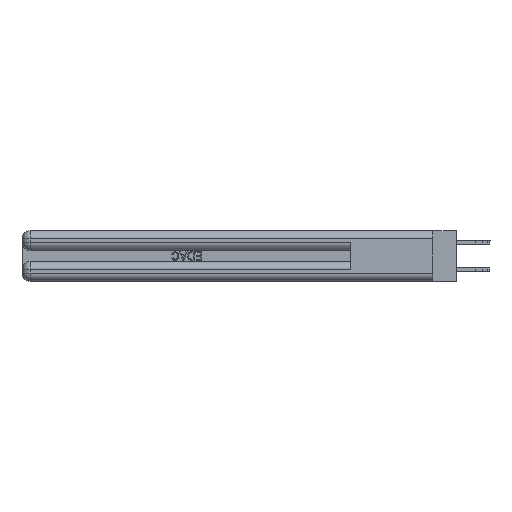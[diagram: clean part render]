
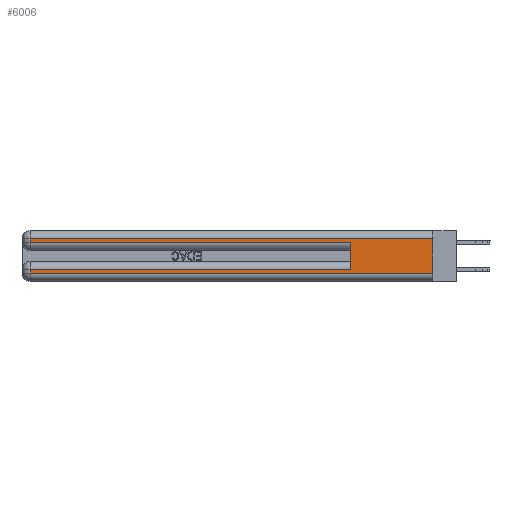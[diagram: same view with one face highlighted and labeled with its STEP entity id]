
A CAD part, left-side view. The second image highlights one B-rep face of the part: STEP entity #6006.
In plain terms, the highlighted planar face has unit normal (-1, 0, 0).
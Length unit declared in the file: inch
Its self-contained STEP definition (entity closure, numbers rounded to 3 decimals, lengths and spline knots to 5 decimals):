
#216 = EDGE_CURVE ( 'NONE', #25626, #29858, #14282, .T. ) ;
#694 = LINE ( 'NONE', #27844, #16419 ) ;
#1438 = VERTEX_POINT ( 'NONE', #34184 ) ;
#1542 = AXIS2_PLACEMENT_3D ( 'NONE', #35377, #20176, #5460 ) ;
#1654 = VERTEX_POINT ( 'NONE', #16338 ) ;
#1658 = CARTESIAN_POINT ( 'NONE',  ( 0., 2.94, 0.37 ) ) ;
#1800 = DIRECTION ( 'NONE',  ( 0., 0., -1. ) ) ;
#2630 = ORIENTED_EDGE ( 'NONE', *, *, #3906, .T. ) ;
#3806 = LINE ( 'NONE', #1658, #14897 ) ;
#3906 = EDGE_CURVE ( 'NONE', #13565, #19742, #37265, .T. ) ;
#4941 = VECTOR ( 'NONE', #24562, 39.37008 ) ;
#5460 = DIRECTION ( 'NONE',  ( 0., 0., -1. ) ) ;
#5715 = VERTEX_POINT ( 'NONE', #21831 ) ;
#5845 = PLANE ( 'NONE',  #1542 ) ;
#6006 = ADVANCED_FACE ( 'NONE', ( #12161 ), #5845, .F. ) ;
#6281 = CARTESIAN_POINT ( 'NONE',  ( 0., 0., 0.285 ) ) ;
#6448 = VECTOR ( 'NONE', #24419, 39.37008 ) ;
#8219 = VECTOR ( 'NONE', #12446, 39.37008 ) ;
#8878 = CARTESIAN_POINT ( 'NONE',  ( 0., 0., 0.06 ) ) ;
#10193 = ORIENTED_EDGE ( 'NONE', *, *, #15186, .T. ) ;
#12161 = FACE_OUTER_BOUND ( 'NONE', #26628, .T. ) ;
#12446 = DIRECTION ( 'NONE',  ( 0., 0., 1. ) ) ;
#13147 = CARTESIAN_POINT ( 'NONE',  ( 0., 0., 0.085 ) ) ;
#13565 = VERTEX_POINT ( 'NONE', #37976 ) ;
#14282 = LINE ( 'NONE', #33454, #6448 ) ;
#14897 = VECTOR ( 'NONE', #1800, 39.37008 ) ;
#15186 = EDGE_CURVE ( 'NONE', #5715, #13565, #16527, .T. ) ;
#15385 = LINE ( 'NONE', #28747, #20918 ) ;
#16338 = CARTESIAN_POINT ( 'NONE',  ( 0., 2.94, 0.085 ) ) ;
#16419 = VECTOR ( 'NONE', #36377, 39.37008 ) ;
#16527 = LINE ( 'NONE', #30966, #19315 ) ;
#18201 = ORIENTED_EDGE ( 'NONE', *, *, #23829, .T. ) ;
#19315 = VECTOR ( 'NONE', #25008, 39.37008 ) ;
#19742 = VERTEX_POINT ( 'NONE', #24199 ) ;
#20176 = DIRECTION ( 'NONE',  ( 1., 0., 0. ) ) ;
#20468 = EDGE_CURVE ( 'NONE', #1438, #1654, #28653, .T. ) ;
#20918 = VECTOR ( 'NONE', #28866, 39.37008 ) ;
#21831 = CARTESIAN_POINT ( 'NONE',  ( 0., 2.94, 0.31 ) ) ;
#22655 = EDGE_CURVE ( 'NONE', #1438, #19742, #25727, .T. ) ;
#22843 = ORIENTED_EDGE ( 'NONE', *, *, #20468, .T. ) ;
#23829 = EDGE_CURVE ( 'NONE', #33414, #29858, #694, .T. ) ;
#24199 = CARTESIAN_POINT ( 'NONE',  ( 0., 0.6, 0.285 ) ) ;
#24371 = ORIENTED_EDGE ( 'NONE', *, *, #22655, .F. ) ;
#24419 = DIRECTION ( 'NONE',  ( 0., 0., -1. ) ) ;
#24562 = DIRECTION ( 'NONE',  ( 0., -1., 0. ) ) ;
#25008 = DIRECTION ( 'NONE',  ( 0., 0., -1. ) ) ;
#25128 = DIRECTION ( 'NONE',  ( 0., 1., 0. ) ) ;
#25626 = VERTEX_POINT ( 'NONE', #28574 ) ;
#25727 = LINE ( 'NONE', #33330, #8219 ) ;
#26342 = EDGE_CURVE ( 'NONE', #25626, #5715, #15385, .T. ) ;
#26628 = EDGE_LOOP ( 'NONE', ( #29538, #35491, #10193, #2630, #24371, #22843, #37061, #18201 ) ) ;
#27742 = VECTOR ( 'NONE', #25128, 39.37008 ) ;
#27844 = CARTESIAN_POINT ( 'NONE',  ( 0., 0., 0.06 ) ) ;
#27931 = EDGE_CURVE ( 'NONE', #1654, #33414, #3806, .T. ) ;
#28574 = CARTESIAN_POINT ( 'NONE',  ( 0., 0., 0.31 ) ) ;
#28653 = LINE ( 'NONE', #13147, #27742 ) ;
#28747 = CARTESIAN_POINT ( 'NONE',  ( 0., 0., 0.31 ) ) ;
#28866 = DIRECTION ( 'NONE',  ( 0., 1., 0. ) ) ;
#29538 = ORIENTED_EDGE ( 'NONE', *, *, #216, .F. ) ;
#29858 = VERTEX_POINT ( 'NONE', #8878 ) ;
#30966 = CARTESIAN_POINT ( 'NONE',  ( 0., 2.94, 0.37 ) ) ;
#32066 = CARTESIAN_POINT ( 'NONE',  ( 0., 2.94, 0.06 ) ) ;
#33330 = CARTESIAN_POINT ( 'NONE',  ( 0., 0.6, 0.145 ) ) ;
#33414 = VERTEX_POINT ( 'NONE', #32066 ) ;
#33454 = CARTESIAN_POINT ( 'NONE',  ( 0., 0., 0.37 ) ) ;
#34184 = CARTESIAN_POINT ( 'NONE',  ( 0., 0.6, 0.085 ) ) ;
#35377 = CARTESIAN_POINT ( 'NONE',  ( 0., 0., 0.37 ) ) ;
#35491 = ORIENTED_EDGE ( 'NONE', *, *, #26342, .T. ) ;
#36377 = DIRECTION ( 'NONE',  ( 0., -1., 0. ) ) ;
#37061 = ORIENTED_EDGE ( 'NONE', *, *, #27931, .T. ) ;
#37265 = LINE ( 'NONE', #6281, #4941 ) ;
#37976 = CARTESIAN_POINT ( 'NONE',  ( 0., 2.94, 0.285 ) ) ;
